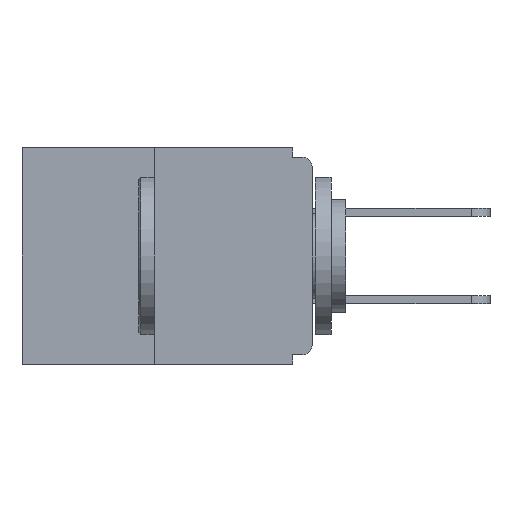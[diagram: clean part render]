
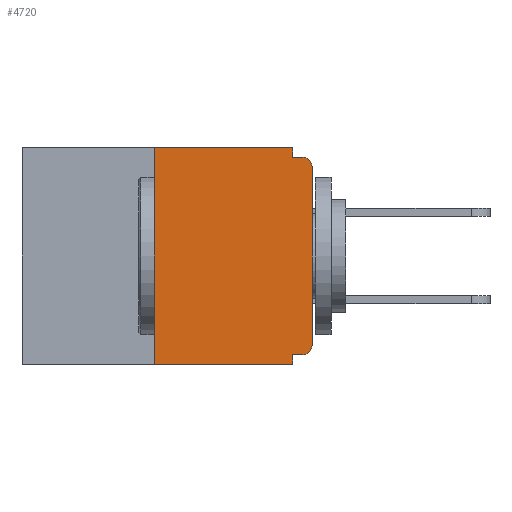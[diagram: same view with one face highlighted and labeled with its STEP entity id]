
A CAD part, left-side view. The second image highlights one B-rep face of the part: STEP entity #4720.
In plain terms, the highlighted planar face has unit normal (-1, 0, 0).
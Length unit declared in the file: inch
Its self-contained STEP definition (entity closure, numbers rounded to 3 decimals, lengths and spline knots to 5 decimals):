
#130 = VERTEX_POINT ( 'NONE', #3139 ) ;
#142 = CARTESIAN_POINT ( 'NONE',  ( 0., 0., -0.015 ) ) ;
#366 = DIRECTION ( 'NONE',  ( -1., 0., 0. ) ) ;
#732 = VERTEX_POINT ( 'NONE', #7534 ) ;
#1049 = ORIENTED_EDGE ( 'NONE', *, *, #12855, .T. ) ;
#1300 = VECTOR ( 'NONE', #8968, 39.37008 ) ;
#1451 = ORIENTED_EDGE ( 'NONE', *, *, #10394, .T. ) ;
#2179 = LINE ( 'NONE', #5555, #2826 ) ;
#2302 = CARTESIAN_POINT ( 'NONE',  ( 0., 0.25, 0. ) ) ;
#2359 = CARTESIAN_POINT ( 'NONE',  ( 0., 0.25, -0.343 ) ) ;
#2571 = CARTESIAN_POINT ( 'NONE',  ( 0., 0.015, -0.015 ) ) ;
#2724 = EDGE_CURVE ( 'NONE', #6480, #3700, #6934, .T. ) ;
#2826 = VECTOR ( 'NONE', #10514, 39.37008 ) ;
#3011 = DIRECTION ( 'NONE',  ( 0., -1., 0. ) ) ;
#3051 = VECTOR ( 'NONE', #8255, 39.37008 ) ;
#3139 = CARTESIAN_POINT ( 'NONE',  ( 0., 0.031, -0.328 ) ) ;
#3161 = ORIENTED_EDGE ( 'NONE', *, *, #2724, .F. ) ;
#3700 = VERTEX_POINT ( 'NONE', #8281 ) ;
#3886 = ORIENTED_EDGE ( 'NONE', *, *, #12271, .F. ) ;
#3899 = CARTESIAN_POINT ( 'NONE',  ( 0., 0.015, -0.313 ) ) ;
#3935 = CARTESIAN_POINT ( 'NONE',  ( 0., 0., 0. ) ) ;
#4069 = FACE_OUTER_BOUND ( 'NONE', #5860, .T. ) ;
#4160 = VERTEX_POINT ( 'NONE', #11583 ) ;
#4455 = ORIENTED_EDGE ( 'NONE', *, *, #5270, .F. ) ;
#4504 = AXIS2_PLACEMENT_3D ( 'NONE', #8306, #366, #11346 ) ;
#4704 = CIRCLE ( 'NONE', #6360, 0.015 ) ;
#4720 = ADVANCED_FACE ( 'NONE', ( #4069 ), #5386, .F. ) ;
#4779 = CARTESIAN_POINT ( 'NONE',  ( 0., 0.46, -0.343 ) ) ;
#4824 = LINE ( 'NONE', #6086, #9624 ) ;
#4844 = CARTESIAN_POINT ( 'NONE',  ( 0., 0.031, -0.343 ) ) ;
#5075 = EDGE_CURVE ( 'NONE', #7236, #4160, #7290, .T. ) ;
#5085 = CARTESIAN_POINT ( 'NONE',  ( 0., 0.46, 0. ) ) ;
#5270 = EDGE_CURVE ( 'NONE', #3700, #7236, #11084, .T. ) ;
#5386 = PLANE ( 'NONE',  #10436 ) ;
#5458 = VECTOR ( 'NONE', #3011, 39.37008 ) ;
#5555 = CARTESIAN_POINT ( 'NONE',  ( 0., 0.031, -0.343 ) ) ;
#5860 = EDGE_LOOP ( 'NONE', ( #4455, #3161, #11682, #11049, #6202, #12034, #1451, #1049, #3886, #9890 ) ) ;
#6046 = LINE ( 'NONE', #4779, #8218 ) ;
#6086 = CARTESIAN_POINT ( 'NONE',  ( 0., 0., -0.328 ) ) ;
#6202 = ORIENTED_EDGE ( 'NONE', *, *, #7029, .F. ) ;
#6360 = AXIS2_PLACEMENT_3D ( 'NONE', #3899, #8705, #11884 ) ;
#6480 = VERTEX_POINT ( 'NONE', #2359 ) ;
#6651 = VERTEX_POINT ( 'NONE', #7523 ) ;
#6833 = EDGE_CURVE ( 'NONE', #6480, #7453, #6046, .T. ) ;
#6846 = VECTOR ( 'NONE', #10730, 39.37008 ) ;
#6934 = LINE ( 'NONE', #2302, #3051 ) ;
#7029 = EDGE_CURVE ( 'NONE', #6651, #130, #4824, .T. ) ;
#7236 = VERTEX_POINT ( 'NONE', #12306 ) ;
#7290 = LINE ( 'NONE', #11664, #6846 ) ;
#7453 = VERTEX_POINT ( 'NONE', #4844 ) ;
#7468 = VERTEX_POINT ( 'NONE', #7779 ) ;
#7523 = CARTESIAN_POINT ( 'NONE',  ( 0., 0.015, -0.328 ) ) ;
#7534 = CARTESIAN_POINT ( 'NONE',  ( 0., 0., -0.03 ) ) ;
#7779 = CARTESIAN_POINT ( 'NONE',  ( 0., 0., -0.313 ) ) ;
#8157 = VERTEX_POINT ( 'NONE', #2571 ) ;
#8218 = VECTOR ( 'NONE', #12792, 39.37008 ) ;
#8255 = DIRECTION ( 'NONE',  ( 0., 0., 1. ) ) ;
#8281 = CARTESIAN_POINT ( 'NONE',  ( 0., 0.25, 0. ) ) ;
#8306 = CARTESIAN_POINT ( 'NONE',  ( 0., 0.015, -0.03 ) ) ;
#8505 = CARTESIAN_POINT ( 'NONE',  ( 0., 0.46, 0. ) ) ;
#8705 = DIRECTION ( 'NONE',  ( -1., 0., 0. ) ) ;
#8966 = LINE ( 'NONE', #142, #1300 ) ;
#8968 = DIRECTION ( 'NONE',  ( 0., -1., 0. ) ) ;
#9549 = LINE ( 'NONE', #3935, #10658 ) ;
#9624 = VECTOR ( 'NONE', #11129, 39.37008 ) ;
#9890 = ORIENTED_EDGE ( 'NONE', *, *, #5075, .F. ) ;
#10394 = EDGE_CURVE ( 'NONE', #7468, #732, #9549, .T. ) ;
#10436 = AXIS2_PLACEMENT_3D ( 'NONE', #8505, #11539, #11360 ) ;
#10514 = DIRECTION ( 'NONE',  ( 0., 0., -1. ) ) ;
#10658 = VECTOR ( 'NONE', #10822, 39.37008 ) ;
#10730 = DIRECTION ( 'NONE',  ( 0., 0., -1. ) ) ;
#10822 = DIRECTION ( 'NONE',  ( 0., 0., 1. ) ) ;
#11049 = ORIENTED_EDGE ( 'NONE', *, *, #11308, .F. ) ;
#11084 = LINE ( 'NONE', #5085, #5458 ) ;
#11129 = DIRECTION ( 'NONE',  ( 0., 1., 0. ) ) ;
#11308 = EDGE_CURVE ( 'NONE', #130, #7453, #2179, .T. ) ;
#11346 = DIRECTION ( 'NONE',  ( 0., 0., -1. ) ) ;
#11360 = DIRECTION ( 'NONE',  ( 0., 0., -1. ) ) ;
#11443 = EDGE_CURVE ( 'NONE', #6651, #7468, #4704, .T. ) ;
#11539 = DIRECTION ( 'NONE',  ( 1., 0., 0. ) ) ;
#11583 = CARTESIAN_POINT ( 'NONE',  ( 0., 0.031, -0.015 ) ) ;
#11664 = CARTESIAN_POINT ( 'NONE',  ( 0., 0.031, 0. ) ) ;
#11682 = ORIENTED_EDGE ( 'NONE', *, *, #6833, .T. ) ;
#11884 = DIRECTION ( 'NONE',  ( 0., 0., -1. ) ) ;
#12034 = ORIENTED_EDGE ( 'NONE', *, *, #11443, .T. ) ;
#12271 = EDGE_CURVE ( 'NONE', #4160, #8157, #8966, .T. ) ;
#12306 = CARTESIAN_POINT ( 'NONE',  ( 0., 0.031, 0. ) ) ;
#12369 = CIRCLE ( 'NONE', #4504, 0.015 ) ;
#12792 = DIRECTION ( 'NONE',  ( 0., -1., 0. ) ) ;
#12855 = EDGE_CURVE ( 'NONE', #732, #8157, #12369, .T. ) ;
